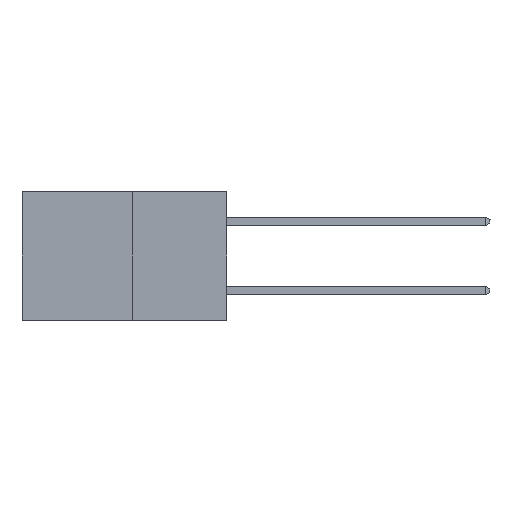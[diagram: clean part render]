
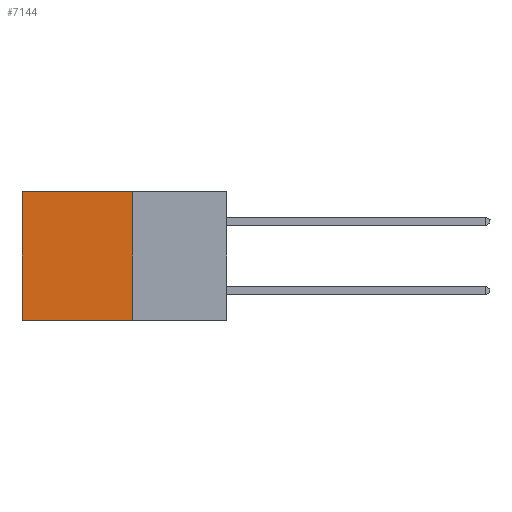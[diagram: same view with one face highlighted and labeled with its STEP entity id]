
A CAD part, left-side view. The second image highlights one B-rep face of the part: STEP entity #7144.
In plain terms, the highlighted planar face has unit normal (-1, 0, 0).
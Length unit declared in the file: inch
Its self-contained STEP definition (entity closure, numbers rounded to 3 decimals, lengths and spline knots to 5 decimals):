
#856 = CARTESIAN_POINT ( 'NONE',  ( 0.277, 0.27, 0. ) ) ;
#1679 = VECTOR ( 'NONE', #9350, 39.37008 ) ;
#2328 = AXIS2_PLACEMENT_3D ( 'NONE', #15161, #14665, #14627 ) ;
#2477 = DIRECTION ( 'NONE',  ( 0., 1., 0. ) ) ;
#3023 = VERTEX_POINT ( 'NONE', #12001 ) ;
#3039 = CARTESIAN_POINT ( 'NONE',  ( 0.277, 0.59, -0.37 ) ) ;
#3459 = ORIENTED_EDGE ( 'NONE', *, *, #14141, .T. ) ;
#3818 = ORIENTED_EDGE ( 'NONE', *, *, #16505, .F. ) ;
#4308 = VERTEX_POINT ( 'NONE', #16586 ) ;
#4378 = VECTOR ( 'NONE', #5285, 39.37008 ) ;
#5285 = DIRECTION ( 'NONE',  ( 0., 0., -1. ) ) ;
#5315 = LINE ( 'NONE', #14630, #1679 ) ;
#5475 = CARTESIAN_POINT ( 'NONE',  ( 0.277, 0.27, -0.37 ) ) ;
#5824 = LINE ( 'NONE', #3039, #8999 ) ;
#6413 = EDGE_CURVE ( 'NONE', #13177, #4308, #11625, .T. ) ;
#7144 = ADVANCED_FACE ( 'NONE', ( #14072 ), #15826, .F. ) ;
#7851 = ORIENTED_EDGE ( 'NONE', *, *, #6413, .F. ) ;
#8468 = DIRECTION ( 'NONE',  ( 0., 0., -1. ) ) ;
#8999 = VECTOR ( 'NONE', #8468, 39.37008 ) ;
#9350 = DIRECTION ( 'NONE',  ( 0., 1., 0. ) ) ;
#9372 = LINE ( 'NONE', #12012, #12522 ) ;
#11625 = LINE ( 'NONE', #5475, #4378 ) ;
#12001 = CARTESIAN_POINT ( 'NONE',  ( 0.277, 0.59, 0. ) ) ;
#12012 = CARTESIAN_POINT ( 'NONE',  ( 0.277, 0.27, 0. ) ) ;
#12522 = VECTOR ( 'NONE', #2477, 39.37008 ) ;
#13177 = VERTEX_POINT ( 'NONE', #856 ) ;
#13771 = ORIENTED_EDGE ( 'NONE', *, *, #16487, .T. ) ;
#14072 = FACE_OUTER_BOUND ( 'NONE', #14286, .T. ) ;
#14141 = EDGE_CURVE ( 'NONE', #3023, #16143, #5824, .T. ) ;
#14286 = EDGE_LOOP ( 'NONE', ( #3459, #3818, #7851, #13771 ) ) ;
#14627 = DIRECTION ( 'NONE',  ( 0., 0., -1. ) ) ;
#14630 = CARTESIAN_POINT ( 'NONE',  ( 0.277, 0.27, -0.37 ) ) ;
#14665 = DIRECTION ( 'NONE',  ( 1., 0., 0. ) ) ;
#15161 = CARTESIAN_POINT ( 'NONE',  ( 0.277, 0.27, -0.37 ) ) ;
#15826 = PLANE ( 'NONE',  #2328 ) ;
#16143 = VERTEX_POINT ( 'NONE', #16593 ) ;
#16487 = EDGE_CURVE ( 'NONE', #13177, #3023, #9372, .T. ) ;
#16505 = EDGE_CURVE ( 'NONE', #4308, #16143, #5315, .T. ) ;
#16586 = CARTESIAN_POINT ( 'NONE',  ( 0.277, 0.27, -0.37 ) ) ;
#16593 = CARTESIAN_POINT ( 'NONE',  ( 0.277, 0.59, -0.37 ) ) ;
